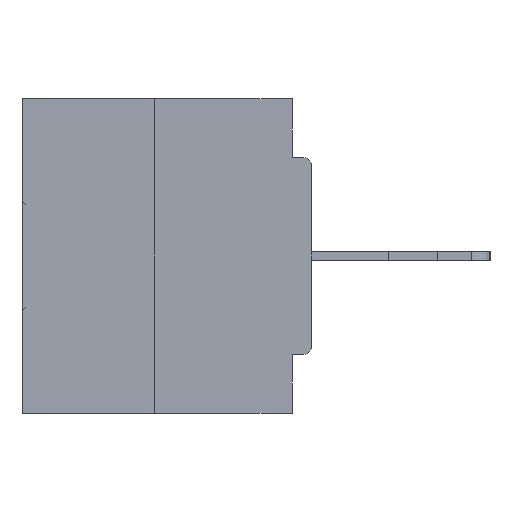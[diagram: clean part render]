
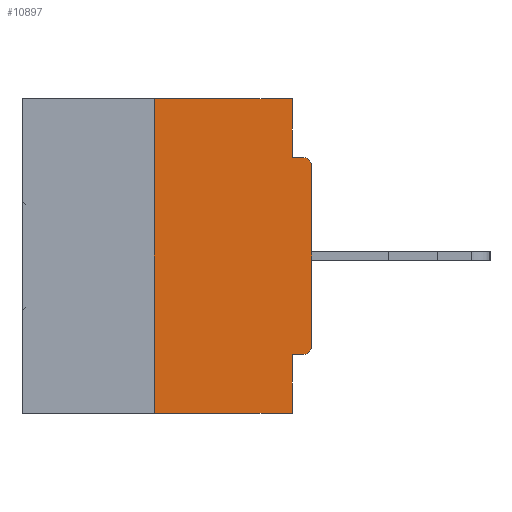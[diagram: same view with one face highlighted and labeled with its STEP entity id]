
A CAD part, left-side view. The second image highlights one B-rep face of the part: STEP entity #10897.
In plain terms, the highlighted planar face has unit normal (-1, 0, 0).
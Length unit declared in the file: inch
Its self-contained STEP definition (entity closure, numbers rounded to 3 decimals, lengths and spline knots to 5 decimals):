
#23 = VERTEX_POINT ( 'NONE', #37015 ) ;
#323 = DIRECTION ( 'NONE',  ( 0., 0., -1. ) ) ;
#1428 = EDGE_CURVE ( 'NONE', #22770, #1935, #24747, .T. ) ;
#1565 = CARTESIAN_POINT ( 'NONE',  ( 0., 0.031, -0.5 ) ) ;
#1935 = VERTEX_POINT ( 'NONE', #25545 ) ;
#1960 = ORIENTED_EDGE ( 'NONE', *, *, #31020, .T. ) ;
#3041 = VERTEX_POINT ( 'NONE', #9542 ) ;
#3087 = PLANE ( 'NONE',  #36194 ) ;
#4666 = DIRECTION ( 'NONE',  ( 0., -1., 0. ) ) ;
#5063 = EDGE_CURVE ( 'NONE', #19473, #13192, #36657, .T. ) ;
#5925 = DIRECTION ( 'NONE',  ( 1., 0., 0. ) ) ;
#6077 = LINE ( 'NONE', #17245, #22434 ) ;
#6229 = VECTOR ( 'NONE', #4666, 39.37008 ) ;
#6342 = DIRECTION ( 'NONE',  ( 0., -1., 0. ) ) ;
#7547 = LINE ( 'NONE', #16263, #17810 ) ;
#7735 = LINE ( 'NONE', #16432, #13932 ) ;
#7766 = CARTESIAN_POINT ( 'NONE',  ( 0., 0., -0.1085 ) ) ;
#7882 = LINE ( 'NONE', #31116, #30945 ) ;
#8159 = DIRECTION ( 'NONE',  ( 0., -1., 0. ) ) ;
#8772 = VERTEX_POINT ( 'NONE', #33073 ) ;
#8906 = AXIS2_PLACEMENT_3D ( 'NONE', #19453, #36960, #30750 ) ;
#9542 = CARTESIAN_POINT ( 'NONE',  ( 0., 0.25, -0.5 ) ) ;
#9747 = ORIENTED_EDGE ( 'NONE', *, *, #21681, .F. ) ;
#10580 = VECTOR ( 'NONE', #323, 39.37008 ) ;
#10764 = DIRECTION ( 'NONE',  ( 0., 0., 1. ) ) ;
#10810 = DIRECTION ( 'NONE',  ( 0., 1., 0. ) ) ;
#10897 = ADVANCED_FACE ( 'NONE', ( #31238 ), #3087, .F. ) ;
#11026 = CARTESIAN_POINT ( 'NONE',  ( 0., 0.46, 0. ) ) ;
#11213 = CARTESIAN_POINT ( 'NONE',  ( 0., 0.031, -0.4065 ) ) ;
#11256 = EDGE_CURVE ( 'NONE', #1935, #19473, #7735, .T. ) ;
#12156 = VERTEX_POINT ( 'NONE', #11213 ) ;
#12432 = LINE ( 'NONE', #15461, #10580 ) ;
#12647 = ORIENTED_EDGE ( 'NONE', *, *, #20337, .F. ) ;
#13192 = VERTEX_POINT ( 'NONE', #26487 ) ;
#13932 = VECTOR ( 'NONE', #10764, 39.37008 ) ;
#15461 = CARTESIAN_POINT ( 'NONE',  ( 0., 0.031, 0. ) ) ;
#15713 = ORIENTED_EDGE ( 'NONE', *, *, #5063, .T. ) ;
#16263 = CARTESIAN_POINT ( 'NONE',  ( 0., 0.25, 0. ) ) ;
#16432 = CARTESIAN_POINT ( 'NONE',  ( 0., 0., 0. ) ) ;
#17245 = CARTESIAN_POINT ( 'NONE',  ( 0., 0.46, -0.5 ) ) ;
#17810 = VECTOR ( 'NONE', #18078, 39.37008 ) ;
#18078 = DIRECTION ( 'NONE',  ( 0., 0., 1. ) ) ;
#18326 = ORIENTED_EDGE ( 'NONE', *, *, #11256, .T. ) ;
#19453 = CARTESIAN_POINT ( 'NONE',  ( 0., 0.015, -0.1085 ) ) ;
#19473 = VERTEX_POINT ( 'NONE', #7766 ) ;
#19527 = LINE ( 'NONE', #36669, #24450 ) ;
#20337 = EDGE_CURVE ( 'NONE', #23, #13192, #21517, .T. ) ;
#21517 = LINE ( 'NONE', #24160, #6229 ) ;
#21681 = EDGE_CURVE ( 'NONE', #22770, #12156, #19527, .T. ) ;
#22260 = EDGE_CURVE ( 'NONE', #25800, #23, #12432, .T. ) ;
#22368 = CARTESIAN_POINT ( 'NONE',  ( 0., 0.031, 0. ) ) ;
#22434 = VECTOR ( 'NONE', #8159, 39.37008 ) ;
#22770 = VERTEX_POINT ( 'NONE', #32909 ) ;
#24160 = CARTESIAN_POINT ( 'NONE',  ( 0., 0., -0.0935 ) ) ;
#24450 = VECTOR ( 'NONE', #10810, 39.37008 ) ;
#24699 = CARTESIAN_POINT ( 'NONE',  ( 0., 0.015, -0.3915 ) ) ;
#24701 = ORIENTED_EDGE ( 'NONE', *, *, #36392, .F. ) ;
#24747 = CIRCLE ( 'NONE', #30100, 0.015 ) ;
#25449 = DIRECTION ( 'NONE',  ( 0., 0., -1. ) ) ;
#25507 = DIRECTION ( 'NONE',  ( 0., 0., -1. ) ) ;
#25545 = CARTESIAN_POINT ( 'NONE',  ( 0., 0., -0.3915 ) ) ;
#25800 = VERTEX_POINT ( 'NONE', #22368 ) ;
#26487 = CARTESIAN_POINT ( 'NONE',  ( 0., 0.015, -0.0935 ) ) ;
#26503 = ORIENTED_EDGE ( 'NONE', *, *, #34739, .F. ) ;
#28115 = EDGE_CURVE ( 'NONE', #8772, #25800, #29563, .T. ) ;
#28282 = ORIENTED_EDGE ( 'NONE', *, *, #28115, .F. ) ;
#29563 = LINE ( 'NONE', #32199, #35367 ) ;
#30073 = ORIENTED_EDGE ( 'NONE', *, *, #1428, .T. ) ;
#30100 = AXIS2_PLACEMENT_3D ( 'NONE', #24699, #33125, #33509 ) ;
#30750 = DIRECTION ( 'NONE',  ( 0., 0., -1. ) ) ;
#30945 = VECTOR ( 'NONE', #25507, 39.37008 ) ;
#31020 = EDGE_CURVE ( 'NONE', #3041, #34098, #6077, .T. ) ;
#31116 = CARTESIAN_POINT ( 'NONE',  ( 0., 0.031, -0.5 ) ) ;
#31238 = FACE_OUTER_BOUND ( 'NONE', #33256, .T. ) ;
#32199 = CARTESIAN_POINT ( 'NONE',  ( 0., 0.46, 0. ) ) ;
#32909 = CARTESIAN_POINT ( 'NONE',  ( 0., 0.015, -0.4065 ) ) ;
#33073 = CARTESIAN_POINT ( 'NONE',  ( 0., 0.25, 0. ) ) ;
#33125 = DIRECTION ( 'NONE',  ( -1., 0., 0. ) ) ;
#33256 = EDGE_LOOP ( 'NONE', ( #28282, #26503, #1960, #24701, #9747, #30073, #18326, #15713, #12647, #37353 ) ) ;
#33509 = DIRECTION ( 'NONE',  ( 0., 0., -1. ) ) ;
#34098 = VERTEX_POINT ( 'NONE', #1565 ) ;
#34739 = EDGE_CURVE ( 'NONE', #3041, #8772, #7547, .T. ) ;
#35367 = VECTOR ( 'NONE', #6342, 39.37008 ) ;
#36194 = AXIS2_PLACEMENT_3D ( 'NONE', #11026, #5925, #25449 ) ;
#36392 = EDGE_CURVE ( 'NONE', #12156, #34098, #7882, .T. ) ;
#36657 = CIRCLE ( 'NONE', #8906, 0.015 ) ;
#36669 = CARTESIAN_POINT ( 'NONE',  ( 0., 0., -0.4065 ) ) ;
#36960 = DIRECTION ( 'NONE',  ( -1., 0., 0. ) ) ;
#37015 = CARTESIAN_POINT ( 'NONE',  ( 0., 0.031, -0.0935 ) ) ;
#37353 = ORIENTED_EDGE ( 'NONE', *, *, #22260, .F. ) ;
